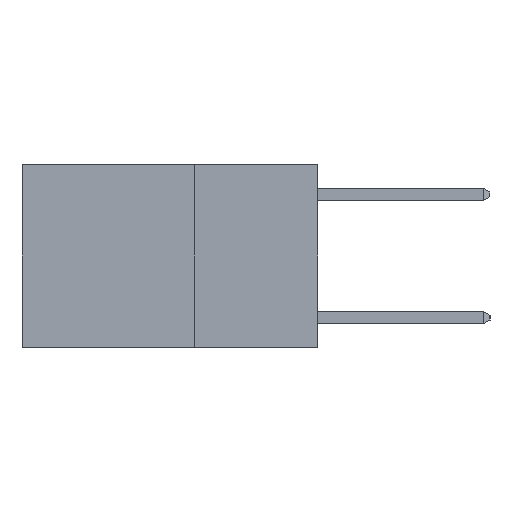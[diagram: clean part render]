
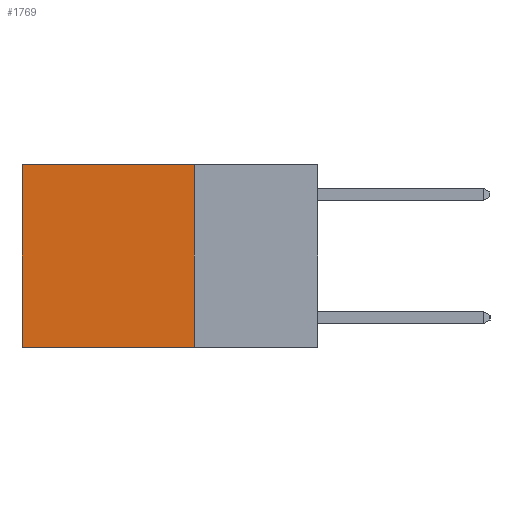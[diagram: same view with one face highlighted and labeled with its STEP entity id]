
A CAD part, left-side view. The second image highlights one B-rep face of the part: STEP entity #1769.
In plain terms, the highlighted planar face has unit normal (-1, 0, 0).
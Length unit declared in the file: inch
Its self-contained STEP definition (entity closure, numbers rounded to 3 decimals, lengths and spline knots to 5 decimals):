
#275 = ORIENTED_EDGE ( 'NONE', *, *, #6673, .T. ) ;
#815 = VERTEX_POINT ( 'NONE', #1938 ) ;
#940 = PLANE ( 'NONE',  #1570 ) ;
#963 = CARTESIAN_POINT ( 'NONE',  ( 0.2625, 0.25, 0. ) ) ;
#1022 = DIRECTION ( 'NONE',  ( 1., 0., 0. ) ) ;
#1167 = ORIENTED_EDGE ( 'NONE', *, *, #3105, .F. ) ;
#1349 = LINE ( 'NONE', #7867, #1569 ) ;
#1569 = VECTOR ( 'NONE', #7864, 39.37008 ) ;
#1570 = AXIS2_PLACEMENT_3D ( 'NONE', #963, #1022, #1733 ) ;
#1733 = DIRECTION ( 'NONE',  ( 0., 0., -1. ) ) ;
#1769 = ADVANCED_FACE ( 'NONE', ( #3829 ), #940, .F. ) ;
#1774 = ORIENTED_EDGE ( 'NONE', *, *, #5983, .T. ) ;
#1938 = CARTESIAN_POINT ( 'NONE',  ( 0.2625, 0.6, 0. ) ) ;
#1994 = VECTOR ( 'NONE', #7532, 39.37008 ) ;
#2147 = VECTOR ( 'NONE', #7311, 39.37008 ) ;
#2179 = EDGE_LOOP ( 'NONE', ( #1774, #1167, #8276, #275 ) ) ;
#2768 = CARTESIAN_POINT ( 'NONE',  ( 0.2625, 0.25, 0. ) ) ;
#2844 = DIRECTION ( 'NONE',  ( 0., 0., -1. ) ) ;
#3003 = CARTESIAN_POINT ( 'NONE',  ( 0.2625, 0.25, 0. ) ) ;
#3027 = VERTEX_POINT ( 'NONE', #8548 ) ;
#3105 = EDGE_CURVE ( 'NONE', #3027, #8277, #1349, .T. ) ;
#3203 = LINE ( 'NONE', #7380, #5753 ) ;
#3578 = LINE ( 'NONE', #3003, #1994 ) ;
#3829 = FACE_OUTER_BOUND ( 'NONE', #2179, .T. ) ;
#4678 = EDGE_CURVE ( 'NONE', #6490, #3027, #7161, .T. ) ;
#5365 = CARTESIAN_POINT ( 'NONE',  ( 0.2625, 0.25, 0. ) ) ;
#5753 = VECTOR ( 'NONE', #2844, 39.37008 ) ;
#5983 = EDGE_CURVE ( 'NONE', #815, #8277, #3203, .T. ) ;
#6490 = VERTEX_POINT ( 'NONE', #5365 ) ;
#6673 = EDGE_CURVE ( 'NONE', #6490, #815, #3578, .T. ) ;
#7161 = LINE ( 'NONE', #2768, #2147 ) ;
#7311 = DIRECTION ( 'NONE',  ( 0., 0., -1. ) ) ;
#7380 = CARTESIAN_POINT ( 'NONE',  ( 0.2625, 0.6, 0. ) ) ;
#7532 = DIRECTION ( 'NONE',  ( 0., 1., 0. ) ) ;
#7830 = CARTESIAN_POINT ( 'NONE',  ( 0.2625, 0.6, -0.37 ) ) ;
#7864 = DIRECTION ( 'NONE',  ( 0., 1., 0. ) ) ;
#7867 = CARTESIAN_POINT ( 'NONE',  ( 0.2625, 0.25, -0.37 ) ) ;
#8276 = ORIENTED_EDGE ( 'NONE', *, *, #4678, .F. ) ;
#8277 = VERTEX_POINT ( 'NONE', #7830 ) ;
#8548 = CARTESIAN_POINT ( 'NONE',  ( 0.2625, 0.25, -0.37 ) ) ;
